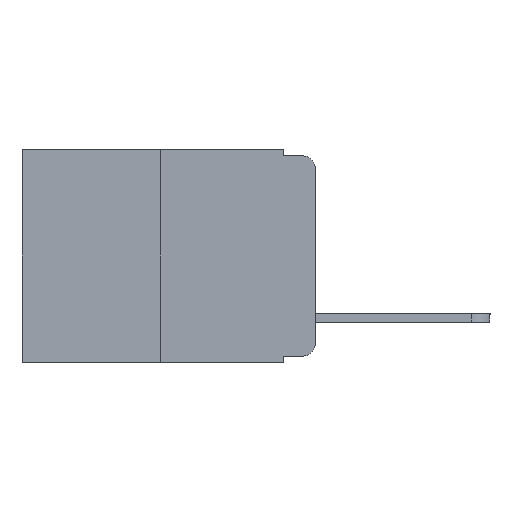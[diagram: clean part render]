
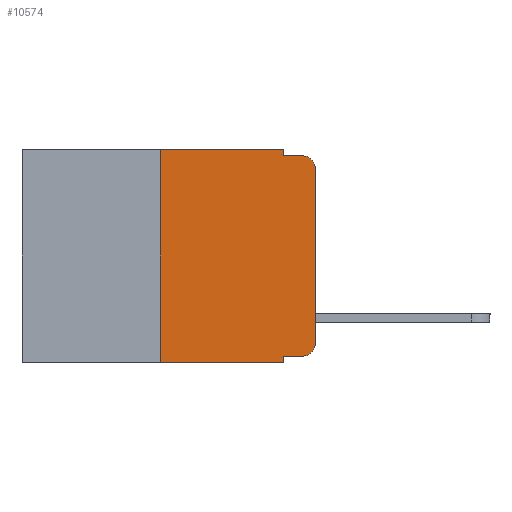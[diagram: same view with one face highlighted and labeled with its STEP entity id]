
A CAD part, left-side view. The second image highlights one B-rep face of the part: STEP entity #10574.
In plain terms, the highlighted planar face has unit normal (-1, 0, 0).
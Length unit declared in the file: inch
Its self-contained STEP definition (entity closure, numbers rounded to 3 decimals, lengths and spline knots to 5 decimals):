
#64 = VECTOR ( 'NONE', #7254, 39.37008 ) ;
#257 = LINE ( 'NONE', #8175, #4893 ) ;
#278 = CARTESIAN_POINT ( 'NONE',  ( 0., 0.051, -0.333 ) ) ;
#638 = DIRECTION ( 'NONE',  ( 0., 0., -1. ) ) ;
#664 = VERTEX_POINT ( 'NONE', #2321 ) ;
#740 = CARTESIAN_POINT ( 'NONE',  ( 0., 0.051, -0.343 ) ) ;
#788 = VECTOR ( 'NONE', #638, 39.37008 ) ;
#893 = VERTEX_POINT ( 'NONE', #10414 ) ;
#1000 = AXIS2_PLACEMENT_3D ( 'NONE', #4909, #9979, #10858 ) ;
#1004 = ORIENTED_EDGE ( 'NONE', *, *, #3074, .T. ) ;
#1126 = VERTEX_POINT ( 'NONE', #6491 ) ;
#1268 = CARTESIAN_POINT ( 'NONE',  ( 0., 0.051, -0.333 ) ) ;
#1339 = CARTESIAN_POINT ( 'NONE',  ( 0., 0.473, 0. ) ) ;
#1511 = DIRECTION ( 'NONE',  ( 0., 0., -1. ) ) ;
#1611 = VERTEX_POINT ( 'NONE', #3736 ) ;
#1737 = CIRCLE ( 'NONE', #7531, 0.02 ) ;
#1973 = ORIENTED_EDGE ( 'NONE', *, *, #10183, .F. ) ;
#2061 = ORIENTED_EDGE ( 'NONE', *, *, #10299, .T. ) ;
#2127 = LINE ( 'NONE', #4955, #9622 ) ;
#2164 = VECTOR ( 'NONE', #7569, 39.37008 ) ;
#2234 = ORIENTED_EDGE ( 'NONE', *, *, #6113, .F. ) ;
#2321 = CARTESIAN_POINT ( 'NONE',  ( 0., 0., -0.313 ) ) ;
#2556 = CARTESIAN_POINT ( 'NONE',  ( 0., 0.02, -0.03 ) ) ;
#2716 = LINE ( 'NONE', #3384, #6200 ) ;
#2974 = DIRECTION ( 'NONE',  ( 0., -1., 0. ) ) ;
#3074 = EDGE_CURVE ( 'NONE', #6867, #5576, #7396, .T. ) ;
#3305 = AXIS2_PLACEMENT_3D ( 'NONE', #6626, #9163, #1511 ) ;
#3308 = EDGE_CURVE ( 'NONE', #10253, #6137, #9261, .T. ) ;
#3341 = LINE ( 'NONE', #8460, #10054 ) ;
#3382 = EDGE_CURVE ( 'NONE', #6867, #6137, #3341, .T. ) ;
#3384 = CARTESIAN_POINT ( 'NONE',  ( 0., 0., 0. ) ) ;
#3463 = VERTEX_POINT ( 'NONE', #8671 ) ;
#3736 = CARTESIAN_POINT ( 'NONE',  ( 0., 0.051, -0.01 ) ) ;
#4202 = CARTESIAN_POINT ( 'NONE',  ( 0., 0.473, -0.343 ) ) ;
#4216 = ORIENTED_EDGE ( 'NONE', *, *, #5940, .F. ) ;
#4315 = EDGE_CURVE ( 'NONE', #5576, #664, #8430, .T. ) ;
#4815 = ORIENTED_EDGE ( 'NONE', *, *, #4870, .F. ) ;
#4863 = PLANE ( 'NONE',  #1000 ) ;
#4870 = EDGE_CURVE ( 'NONE', #1126, #3463, #10025, .T. ) ;
#4893 = VECTOR ( 'NONE', #2974, 39.37008 ) ;
#4909 = CARTESIAN_POINT ( 'NONE',  ( 0., 0.473, 0. ) ) ;
#4955 = CARTESIAN_POINT ( 'NONE',  ( 0., 0.25, 0. ) ) ;
#5173 = ORIENTED_EDGE ( 'NONE', *, *, #3308, .T. ) ;
#5453 = VECTOR ( 'NONE', #10898, 39.37008 ) ;
#5576 = VERTEX_POINT ( 'NONE', #7631 ) ;
#5846 = ORIENTED_EDGE ( 'NONE', *, *, #7945, .T. ) ;
#5909 = DIRECTION ( 'NONE',  ( 0., 0., -1. ) ) ;
#5940 = EDGE_CURVE ( 'NONE', #1611, #10890, #257, .T. ) ;
#5999 = FACE_OUTER_BOUND ( 'NONE', #9896, .T. ) ;
#6113 = EDGE_CURVE ( 'NONE', #3463, #1611, #10252, .T. ) ;
#6137 = VERTEX_POINT ( 'NONE', #740 ) ;
#6200 = VECTOR ( 'NONE', #7659, 39.37008 ) ;
#6248 = ORIENTED_EDGE ( 'NONE', *, *, #3382, .F. ) ;
#6491 = CARTESIAN_POINT ( 'NONE',  ( 0., 0.25, 0. ) ) ;
#6626 = CARTESIAN_POINT ( 'NONE',  ( 0., 0.02, -0.313 ) ) ;
#6867 = VERTEX_POINT ( 'NONE', #278 ) ;
#7005 = DIRECTION ( 'NONE',  ( -1., 0., 0. ) ) ;
#7065 = CARTESIAN_POINT ( 'NONE',  ( 0., 0.02, -0.01 ) ) ;
#7254 = DIRECTION ( 'NONE',  ( 0., -1., 0. ) ) ;
#7396 = LINE ( 'NONE', #1268, #64 ) ;
#7531 = AXIS2_PLACEMENT_3D ( 'NONE', #2556, #7005, #8718 ) ;
#7569 = DIRECTION ( 'NONE',  ( 0., -1., 0. ) ) ;
#7631 = CARTESIAN_POINT ( 'NONE',  ( 0., 0.02, -0.333 ) ) ;
#7659 = DIRECTION ( 'NONE',  ( 0., 0., 1. ) ) ;
#7862 = DIRECTION ( 'NONE',  ( 0., 0., 1. ) ) ;
#7933 = CARTESIAN_POINT ( 'NONE',  ( 0., 0.25, -0.343 ) ) ;
#7945 = EDGE_CURVE ( 'NONE', #664, #893, #2716, .T. ) ;
#8175 = CARTESIAN_POINT ( 'NONE',  ( 0., 0.051, -0.01 ) ) ;
#8430 = CIRCLE ( 'NONE', #3305, 0.02 ) ;
#8460 = CARTESIAN_POINT ( 'NONE',  ( 0., 0.051, 0. ) ) ;
#8671 = CARTESIAN_POINT ( 'NONE',  ( 0., 0.051, 0. ) ) ;
#8718 = DIRECTION ( 'NONE',  ( 0., 0., -1. ) ) ;
#9163 = DIRECTION ( 'NONE',  ( -1., 0., 0. ) ) ;
#9261 = LINE ( 'NONE', #4202, #2164 ) ;
#9622 = VECTOR ( 'NONE', #7862, 39.37008 ) ;
#9896 = EDGE_LOOP ( 'NONE', ( #5846, #2061, #4216, #2234, #4815, #1973, #5173, #6248, #1004, #10747 ) ) ;
#9979 = DIRECTION ( 'NONE',  ( 1., 0., 0. ) ) ;
#10025 = LINE ( 'NONE', #1339, #5453 ) ;
#10054 = VECTOR ( 'NONE', #5909, 39.37008 ) ;
#10133 = CARTESIAN_POINT ( 'NONE',  ( 0., 0.051, 0. ) ) ;
#10183 = EDGE_CURVE ( 'NONE', #10253, #1126, #2127, .T. ) ;
#10252 = LINE ( 'NONE', #10133, #788 ) ;
#10253 = VERTEX_POINT ( 'NONE', #7933 ) ;
#10299 = EDGE_CURVE ( 'NONE', #893, #10890, #1737, .T. ) ;
#10414 = CARTESIAN_POINT ( 'NONE',  ( 0., 0., -0.03 ) ) ;
#10574 = ADVANCED_FACE ( 'NONE', ( #5999 ), #4863, .F. ) ;
#10747 = ORIENTED_EDGE ( 'NONE', *, *, #4315, .T. ) ;
#10858 = DIRECTION ( 'NONE',  ( 0., 0., -1. ) ) ;
#10890 = VERTEX_POINT ( 'NONE', #7065 ) ;
#10898 = DIRECTION ( 'NONE',  ( 0., -1., 0. ) ) ;
